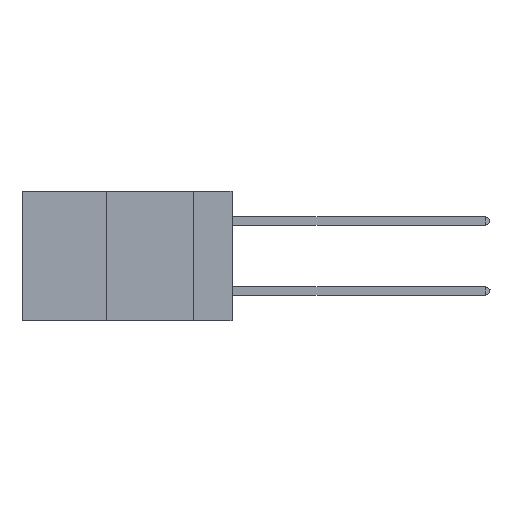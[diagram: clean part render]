
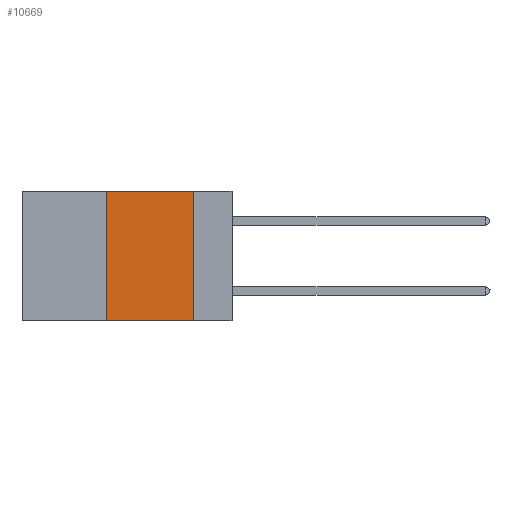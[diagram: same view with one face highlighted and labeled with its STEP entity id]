
A CAD part, left-side view. The second image highlights one B-rep face of the part: STEP entity #10669.
In plain terms, the highlighted planar face has unit normal (-1, 0, 0).
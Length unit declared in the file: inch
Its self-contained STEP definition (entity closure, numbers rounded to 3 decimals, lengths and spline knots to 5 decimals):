
#1420 = DIRECTION ( 'NONE',  ( 0., 0., -1. ) ) ;
#1946 = DIRECTION ( 'NONE',  ( 0., 0., 1. ) ) ;
#3420 = VERTEX_POINT ( 'NONE', #15357 ) ;
#3584 = LINE ( 'NONE', #21089, #13753 ) ;
#3785 = FACE_OUTER_BOUND ( 'NONE', #15616, .T. ) ;
#3924 = DIRECTION ( 'NONE',  ( 0., 0., -1. ) ) ;
#4085 = ORIENTED_EDGE ( 'NONE', *, *, #19769, .F. ) ;
#4755 = VERTEX_POINT ( 'NONE', #7067 ) ;
#4757 = VERTEX_POINT ( 'NONE', #26441 ) ;
#5535 = EDGE_CURVE ( 'NONE', #4757, #19561, #27958, .T. ) ;
#6231 = VECTOR ( 'NONE', #18421, 39.37008 ) ;
#6968 = LINE ( 'NONE', #25034, #6231 ) ;
#7067 = CARTESIAN_POINT ( 'NONE',  ( 0., 0.36, 0. ) ) ;
#7897 = VECTOR ( 'NONE', #1420, 39.37008 ) ;
#10669 = ADVANCED_FACE ( 'NONE', ( #3785 ), #12539, .F. ) ;
#11121 = LINE ( 'NONE', #21756, #13174 ) ;
#12324 = CARTESIAN_POINT ( 'NONE',  ( 0., 0.11, 0. ) ) ;
#12539 = PLANE ( 'NONE',  #21622 ) ;
#13174 = VECTOR ( 'NONE', #1946, 39.37008 ) ;
#13191 = ORIENTED_EDGE ( 'NONE', *, *, #22235, .F. ) ;
#13753 = VECTOR ( 'NONE', #25528, 39.37008 ) ;
#15357 = CARTESIAN_POINT ( 'NONE',  ( 0., 0.36, -0.37 ) ) ;
#15616 = EDGE_LOOP ( 'NONE', ( #16329, #13191, #4085, #27076 ) ) ;
#15720 = EDGE_CURVE ( 'NONE', #3420, #19561, #6968, .T. ) ;
#16329 = ORIENTED_EDGE ( 'NONE', *, *, #5535, .F. ) ;
#16970 = DIRECTION ( 'NONE',  ( 1., 0., 0. ) ) ;
#18421 = DIRECTION ( 'NONE',  ( 0., -1., 0. ) ) ;
#19561 = VERTEX_POINT ( 'NONE', #20627 ) ;
#19769 = EDGE_CURVE ( 'NONE', #3420, #4755, #11121, .T. ) ;
#20627 = CARTESIAN_POINT ( 'NONE',  ( 0., 0.11, -0.37 ) ) ;
#21089 = CARTESIAN_POINT ( 'NONE',  ( 0., 0.6, 0. ) ) ;
#21295 = CARTESIAN_POINT ( 'NONE',  ( 0., 0.6, 0. ) ) ;
#21622 = AXIS2_PLACEMENT_3D ( 'NONE', #21295, #16970, #3924 ) ;
#21756 = CARTESIAN_POINT ( 'NONE',  ( 0., 0.36, 0. ) ) ;
#22235 = EDGE_CURVE ( 'NONE', #4755, #4757, #3584, .T. ) ;
#25034 = CARTESIAN_POINT ( 'NONE',  ( 0., 0.6, -0.37 ) ) ;
#25528 = DIRECTION ( 'NONE',  ( 0., -1., 0. ) ) ;
#26441 = CARTESIAN_POINT ( 'NONE',  ( 0., 0.11, 0. ) ) ;
#27076 = ORIENTED_EDGE ( 'NONE', *, *, #15720, .T. ) ;
#27958 = LINE ( 'NONE', #12324, #7897 ) ;
